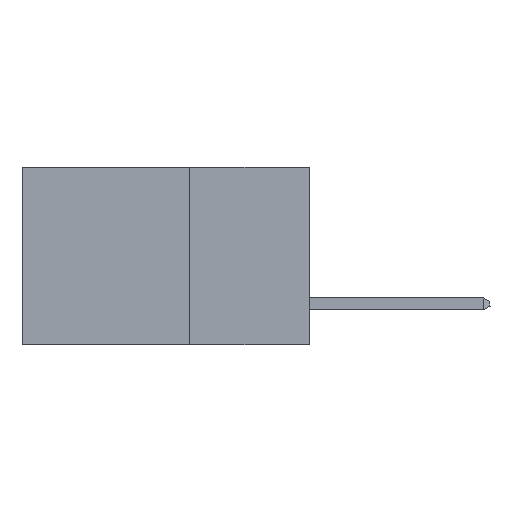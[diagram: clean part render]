
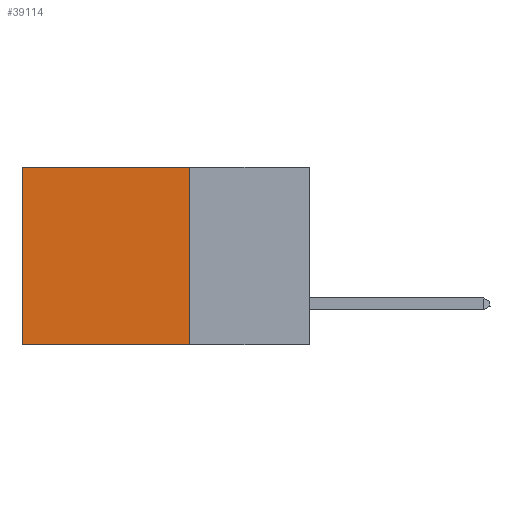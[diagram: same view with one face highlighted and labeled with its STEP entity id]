
A CAD part, left-side view. The second image highlights one B-rep face of the part: STEP entity #39114.
In plain terms, the highlighted planar face has unit normal (-1, 0, 0).
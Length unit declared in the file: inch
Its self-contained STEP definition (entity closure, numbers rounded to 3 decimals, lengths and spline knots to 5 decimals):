
#1375 = LINE ( 'NONE', #20665, #41355 ) ;
#2322 = CARTESIAN_POINT ( 'NONE',  ( 0.2875, 0.6, -0.37 ) ) ;
#5557 = EDGE_CURVE ( 'NONE', #41791, #40273, #9668, .T. ) ;
#8954 = CARTESIAN_POINT ( 'NONE',  ( 0.2875, 0.6, 0. ) ) ;
#9035 = EDGE_LOOP ( 'NONE', ( #10570, #25239, #46722, #32894 ) ) ;
#9668 = LINE ( 'NONE', #14645, #27809 ) ;
#10570 = ORIENTED_EDGE ( 'NONE', *, *, #47930, .T. ) ;
#14645 = CARTESIAN_POINT ( 'NONE',  ( 0.2875, 0.25, 0. ) ) ;
#14817 = DIRECTION ( 'NONE',  ( 0., 0., -1. ) ) ;
#15366 = CARTESIAN_POINT ( 'NONE',  ( 0.2875, 0.25, 0. ) ) ;
#17742 = DIRECTION ( 'NONE',  ( 0., 1., 0. ) ) ;
#20665 = CARTESIAN_POINT ( 'NONE',  ( 0.2875, 0.6, 0. ) ) ;
#23451 = VECTOR ( 'NONE', #26100, 39.37008 ) ;
#23795 = FACE_OUTER_BOUND ( 'NONE', #9035, .T. ) ;
#25150 = AXIS2_PLACEMENT_3D ( 'NONE', #15366, #42427, #46343 ) ;
#25239 = ORIENTED_EDGE ( 'NONE', *, *, #38844, .F. ) ;
#26100 = DIRECTION ( 'NONE',  ( 0., 1., 0. ) ) ;
#27809 = VECTOR ( 'NONE', #14817, 39.37008 ) ;
#28974 = LINE ( 'NONE', #37269, #23451 ) ;
#30524 = EDGE_CURVE ( 'NONE', #41791, #36292, #28974, .T. ) ;
#32894 = ORIENTED_EDGE ( 'NONE', *, *, #30524, .T. ) ;
#34635 = PLANE ( 'NONE',  #25150 ) ;
#36292 = VERTEX_POINT ( 'NONE', #8954 ) ;
#37035 = CARTESIAN_POINT ( 'NONE',  ( 0.2875, 0.25, -0.37 ) ) ;
#37269 = CARTESIAN_POINT ( 'NONE',  ( 0.2875, 0.25, 0. ) ) ;
#38098 = CARTESIAN_POINT ( 'NONE',  ( 0.2875, 0.25, -0.37 ) ) ;
#38844 = EDGE_CURVE ( 'NONE', #40273, #45892, #40834, .T. ) ;
#39114 = ADVANCED_FACE ( 'NONE', ( #23795 ), #34635, .F. ) ;
#40273 = VERTEX_POINT ( 'NONE', #38098 ) ;
#40834 = LINE ( 'NONE', #37035, #46293 ) ;
#41355 = VECTOR ( 'NONE', #47287, 39.37008 ) ;
#41791 = VERTEX_POINT ( 'NONE', #43035 ) ;
#42427 = DIRECTION ( 'NONE',  ( 1., 0., 0. ) ) ;
#43035 = CARTESIAN_POINT ( 'NONE',  ( 0.2875, 0.25, 0. ) ) ;
#45892 = VERTEX_POINT ( 'NONE', #2322 ) ;
#46293 = VECTOR ( 'NONE', #17742, 39.37008 ) ;
#46343 = DIRECTION ( 'NONE',  ( 0., 0., -1. ) ) ;
#46722 = ORIENTED_EDGE ( 'NONE', *, *, #5557, .F. ) ;
#47287 = DIRECTION ( 'NONE',  ( 0., 0., -1. ) ) ;
#47930 = EDGE_CURVE ( 'NONE', #36292, #45892, #1375, .T. ) ;
